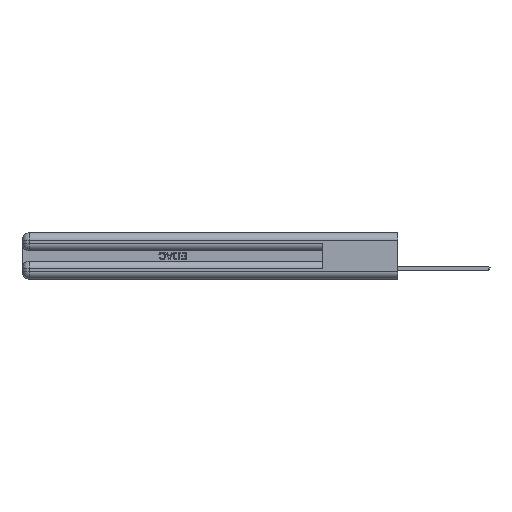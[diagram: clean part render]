
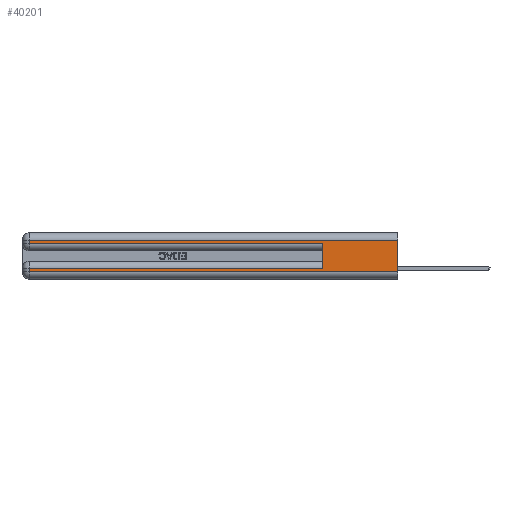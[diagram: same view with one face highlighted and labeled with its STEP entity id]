
A CAD part, left-side view. The second image highlights one B-rep face of the part: STEP entity #40201.
In plain terms, the highlighted planar face has unit normal (-1, 0, 0).
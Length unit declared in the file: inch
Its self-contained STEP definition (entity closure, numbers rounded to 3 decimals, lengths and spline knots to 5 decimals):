
#3044 = VERTEX_POINT ( 'NONE', #38720 ) ;
#3746 = CARTESIAN_POINT ( 'NONE',  ( 0., 0.6, 0.085 ) ) ;
#3755 = DIRECTION ( 'NONE',  ( 1., 0., 0. ) ) ;
#4208 = VECTOR ( 'NONE', #26750, 39.37008 ) ;
#5166 = VERTEX_POINT ( 'NONE', #21717 ) ;
#5920 = ORIENTED_EDGE ( 'NONE', *, *, #26440, .T. ) ;
#6026 = DIRECTION ( 'NONE',  ( 0., 1., 0. ) ) ;
#6359 = CARTESIAN_POINT ( 'NONE',  ( 0., 0., 0.31 ) ) ;
#6451 = DIRECTION ( 'NONE',  ( 0., 0., -1. ) ) ;
#7874 = VECTOR ( 'NONE', #6026, 39.37008 ) ;
#8528 = EDGE_CURVE ( 'NONE', #5166, #30720, #23155, .T. ) ;
#8760 = EDGE_CURVE ( 'NONE', #21636, #22287, #45000, .T. ) ;
#9090 = ORIENTED_EDGE ( 'NONE', *, *, #8760, .T. ) ;
#9552 = LINE ( 'NONE', #48065, #36812 ) ;
#10489 = CARTESIAN_POINT ( 'NONE',  ( 0., 2.94, 0.31 ) ) ;
#10624 = DIRECTION ( 'NONE',  ( 0., 0., -1. ) ) ;
#10954 = CARTESIAN_POINT ( 'NONE',  ( 0., 2.94, 0.37 ) ) ;
#12351 = PLANE ( 'NONE',  #32965 ) ;
#12683 = VERTEX_POINT ( 'NONE', #26652 ) ;
#12696 = DIRECTION ( 'NONE',  ( 0., 0., 1. ) ) ;
#13992 = VECTOR ( 'NONE', #32085, 39.37008 ) ;
#14503 = CARTESIAN_POINT ( 'NONE',  ( 0., 0., 0.085 ) ) ;
#16659 = ORIENTED_EDGE ( 'NONE', *, *, #44236, .T. ) ;
#17043 = EDGE_CURVE ( 'NONE', #21431, #22287, #45551, .T. ) ;
#20359 = CARTESIAN_POINT ( 'NONE',  ( 0., 0., 0.285 ) ) ;
#21196 = DIRECTION ( 'NONE',  ( 0., 0., -1. ) ) ;
#21431 = VERTEX_POINT ( 'NONE', #3746 ) ;
#21636 = VERTEX_POINT ( 'NONE', #26611 ) ;
#21717 = CARTESIAN_POINT ( 'NONE',  ( 0., 2.94, 0.085 ) ) ;
#21970 = ORIENTED_EDGE ( 'NONE', *, *, #8528, .T. ) ;
#22101 = CARTESIAN_POINT ( 'NONE',  ( 0., 0.6, 0.285 ) ) ;
#22287 = VERTEX_POINT ( 'NONE', #22101 ) ;
#22849 = ORIENTED_EDGE ( 'NONE', *, *, #17043, .F. ) ;
#23155 = LINE ( 'NONE', #10954, #41418 ) ;
#23548 = FACE_OUTER_BOUND ( 'NONE', #28361, .T. ) ;
#23551 = LINE ( 'NONE', #14503, #4208 ) ;
#24212 = LINE ( 'NONE', #6359, #7874 ) ;
#24327 = VECTOR ( 'NONE', #6451, 39.37008 ) ;
#24857 = DIRECTION ( 'NONE',  ( 0., -1., 0. ) ) ;
#26440 = EDGE_CURVE ( 'NONE', #30720, #3044, #41432, .T. ) ;
#26611 = CARTESIAN_POINT ( 'NONE',  ( 0., 2.94, 0.285 ) ) ;
#26652 = CARTESIAN_POINT ( 'NONE',  ( 0., 0., 0.31 ) ) ;
#26750 = DIRECTION ( 'NONE',  ( 0., 1., 0. ) ) ;
#27631 = CARTESIAN_POINT ( 'NONE',  ( 0., 0.6, 0.145 ) ) ;
#28087 = DIRECTION ( 'NONE',  ( 0., 0., -1. ) ) ;
#28361 = EDGE_LOOP ( 'NONE', ( #44318, #16659, #33915, #9090, #22849, #46572, #21970, #5920 ) ) ;
#28413 = EDGE_CURVE ( 'NONE', #21431, #5166, #23551, .T. ) ;
#30720 = VERTEX_POINT ( 'NONE', #47359 ) ;
#32085 = DIRECTION ( 'NONE',  ( 0., -1., 0. ) ) ;
#32965 = AXIS2_PLACEMENT_3D ( 'NONE', #39510, #3755, #28087 ) ;
#33496 = VECTOR ( 'NONE', #24857, 39.37008 ) ;
#33915 = ORIENTED_EDGE ( 'NONE', *, *, #35080, .T. ) ;
#34615 = VECTOR ( 'NONE', #12696, 39.37008 ) ;
#35080 = EDGE_CURVE ( 'NONE', #48829, #21636, #38403, .T. ) ;
#36812 = VECTOR ( 'NONE', #21196, 39.37008 ) ;
#38403 = LINE ( 'NONE', #49565, #24327 ) ;
#38720 = CARTESIAN_POINT ( 'NONE',  ( 0., 0., 0.06 ) ) ;
#39342 = CARTESIAN_POINT ( 'NONE',  ( 0., 0., 0.06 ) ) ;
#39510 = CARTESIAN_POINT ( 'NONE',  ( 0., 0., 0.37 ) ) ;
#40201 = ADVANCED_FACE ( 'NONE', ( #23548 ), #12351, .F. ) ;
#41418 = VECTOR ( 'NONE', #10624, 39.37008 ) ;
#41432 = LINE ( 'NONE', #39342, #33496 ) ;
#44236 = EDGE_CURVE ( 'NONE', #12683, #48829, #24212, .T. ) ;
#44318 = ORIENTED_EDGE ( 'NONE', *, *, #45817, .F. ) ;
#45000 = LINE ( 'NONE', #20359, #13992 ) ;
#45551 = LINE ( 'NONE', #27631, #34615 ) ;
#45817 = EDGE_CURVE ( 'NONE', #12683, #3044, #9552, .T. ) ;
#46572 = ORIENTED_EDGE ( 'NONE', *, *, #28413, .T. ) ;
#47359 = CARTESIAN_POINT ( 'NONE',  ( 0., 2.94, 0.06 ) ) ;
#48065 = CARTESIAN_POINT ( 'NONE',  ( 0., 0., 0.37 ) ) ;
#48829 = VERTEX_POINT ( 'NONE', #10489 ) ;
#49565 = CARTESIAN_POINT ( 'NONE',  ( 0., 2.94, 0.37 ) ) ;
